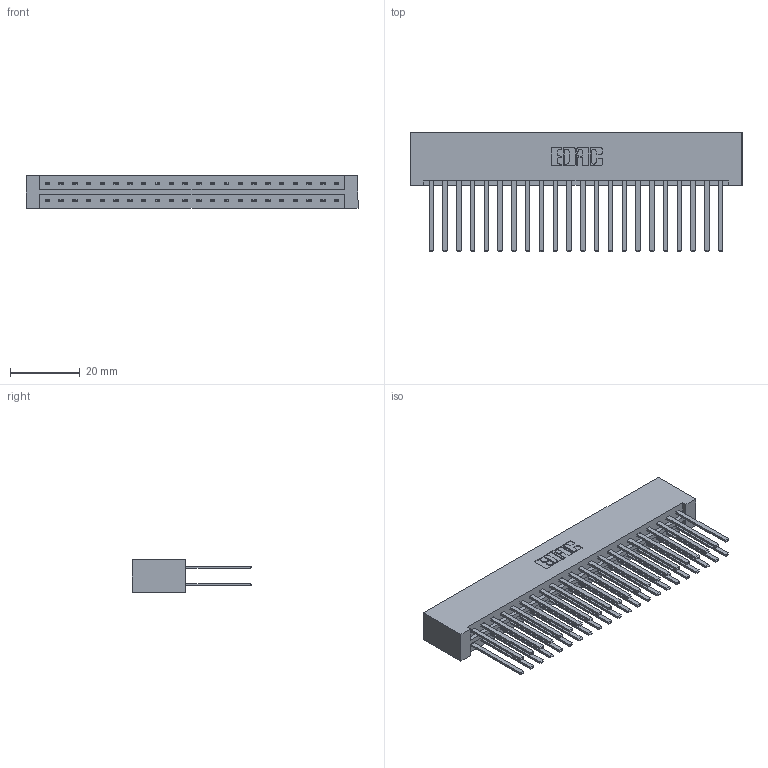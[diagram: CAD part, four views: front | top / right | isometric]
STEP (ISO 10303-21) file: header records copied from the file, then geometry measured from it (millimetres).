
FILE_DESCRIPTION (( 'STEP AP203' ), '1' );
FILE_NAME ('333-044-544-201.STEP', '2018-08-03T21:24:58', ( '' ), ( '' ), 'SwSTEP 2.0', 'SolidWorks 2016', '' );
FILE_SCHEMA (( 'CONFIG_CONTROL_DESIGN' ));
Length unit declared in the file: inch
Products named in the file (3): 333-044-544-201; 333 Part_Lugless; 345-292-001_345-293-144
Assembly tree (45 placements, depth 2):
  333-044-544-201
    333 Part_Lugless
    345-292-001_345-293-144  x44
Bounding box: 95.43 x 34.3 x 9.4 mm (x, y, z)
Volume: 10804.6 mm3; surface area: 14569.1 mm2
Topology: 45 solids, 45 shells, 2130 faces, 6315 edges, 4150 vertices
Faces by surface type: plane 1474, cylinder 656
Entity records: 16279 total; most frequent: CARTESIAN_POINT 2718, ORIENTED_EDGE 2654, DIRECTION 2347, EDGE_CURVE 1327, LINE 1211, VECTOR 1211, VERTEX_POINT 882, AXIS2_PLACEMENT_3D 568
